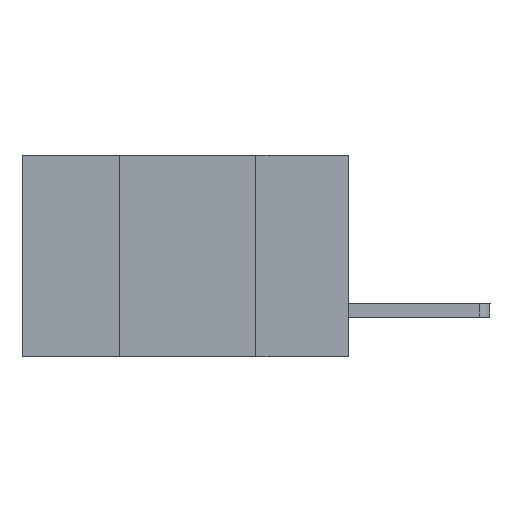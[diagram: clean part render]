
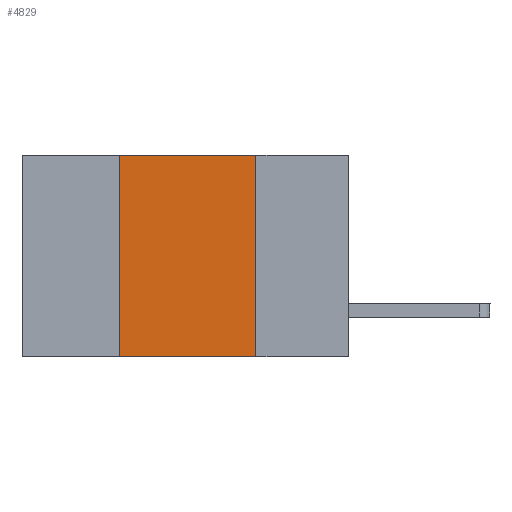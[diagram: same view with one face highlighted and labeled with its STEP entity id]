
A CAD part, left-side view. The second image highlights one B-rep face of the part: STEP entity #4829.
In plain terms, the highlighted planar face has unit normal (-1, 0, 0).
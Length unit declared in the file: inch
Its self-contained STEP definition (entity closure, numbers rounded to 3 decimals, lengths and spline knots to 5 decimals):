
#216 = EDGE_CURVE ( 'NONE', #5213, #3487, #897, .T. ) ;
#265 = VECTOR ( 'NONE', #7434, 39.37008 ) ;
#339 = CARTESIAN_POINT ( 'NONE',  ( 0., 0.6, 0. ) ) ;
#468 = VECTOR ( 'NONE', #1236, 39.37008 ) ;
#761 = EDGE_CURVE ( 'NONE', #2082, #6432, #10001, .T. ) ;
#897 = LINE ( 'NONE', #8240, #265 ) ;
#932 = DIRECTION ( 'NONE',  ( 0., 0., 1. ) ) ;
#1236 = DIRECTION ( 'NONE',  ( 0., -1., 0. ) ) ;
#1815 = LINE ( 'NONE', #8553, #468 ) ;
#1940 = AXIS2_PLACEMENT_3D ( 'NONE', #339, #8342, #8277 ) ;
#2082 = VERTEX_POINT ( 'NONE', #2351 ) ;
#2144 = DIRECTION ( 'NONE',  ( 0., -1., 0. ) ) ;
#2146 = EDGE_CURVE ( 'NONE', #2082, #3487, #9461, .T. ) ;
#2351 = CARTESIAN_POINT ( 'NONE',  ( 0., 0.42, -0.37 ) ) ;
#2511 = VECTOR ( 'NONE', #2144, 39.37008 ) ;
#3392 = ORIENTED_EDGE ( 'NONE', *, *, #2146, .T. ) ;
#3461 = ORIENTED_EDGE ( 'NONE', *, *, #761, .F. ) ;
#3487 = VERTEX_POINT ( 'NONE', #7474 ) ;
#3528 = PLANE ( 'NONE',  #1940 ) ;
#4829 = ADVANCED_FACE ( 'NONE', ( #9942 ), #3528, .F. ) ;
#5015 = CARTESIAN_POINT ( 'NONE',  ( 0., 0.42, -0.37 ) ) ;
#5213 = VERTEX_POINT ( 'NONE', #10040 ) ;
#5773 = CARTESIAN_POINT ( 'NONE',  ( 0., 0.42, 0. ) ) ;
#6432 = VERTEX_POINT ( 'NONE', #5773 ) ;
#6551 = EDGE_LOOP ( 'NONE', ( #6658, #9801, #3461, #3392 ) ) ;
#6658 = ORIENTED_EDGE ( 'NONE', *, *, #216, .F. ) ;
#6739 = VECTOR ( 'NONE', #932, 39.37008 ) ;
#7434 = DIRECTION ( 'NONE',  ( 0., 0., -1. ) ) ;
#7474 = CARTESIAN_POINT ( 'NONE',  ( 0., 0.17, -0.37 ) ) ;
#8240 = CARTESIAN_POINT ( 'NONE',  ( 0., 0.17, -0.37 ) ) ;
#8277 = DIRECTION ( 'NONE',  ( 0., 0., -1. ) ) ;
#8342 = DIRECTION ( 'NONE',  ( 1., 0., 0. ) ) ;
#8553 = CARTESIAN_POINT ( 'NONE',  ( 0., 0.6, 0. ) ) ;
#8784 = EDGE_CURVE ( 'NONE', #6432, #5213, #1815, .T. ) ;
#9461 = LINE ( 'NONE', #10424, #2511 ) ;
#9801 = ORIENTED_EDGE ( 'NONE', *, *, #8784, .F. ) ;
#9942 = FACE_OUTER_BOUND ( 'NONE', #6551, .T. ) ;
#10001 = LINE ( 'NONE', #5015, #6739 ) ;
#10040 = CARTESIAN_POINT ( 'NONE',  ( 0., 0.17, 0. ) ) ;
#10424 = CARTESIAN_POINT ( 'NONE',  ( 0., 0.6, -0.37 ) ) ;
